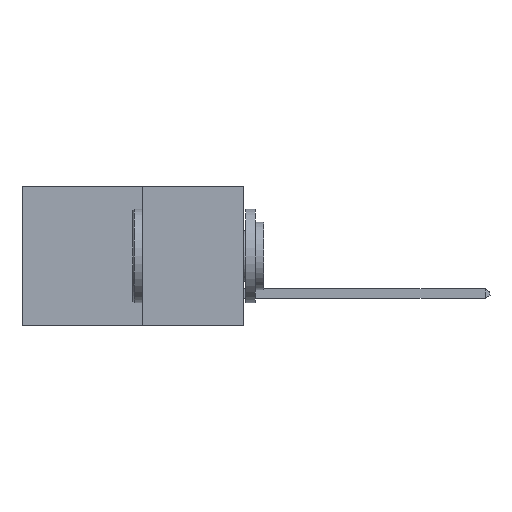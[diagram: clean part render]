
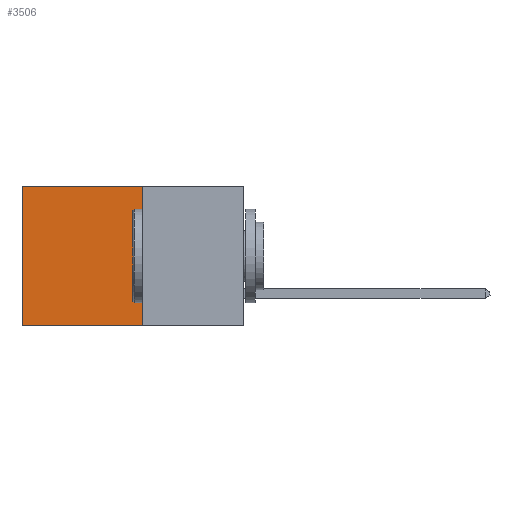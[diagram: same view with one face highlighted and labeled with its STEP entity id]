
A CAD part, left-side view. The second image highlights one B-rep face of the part: STEP entity #3506.
In plain terms, the highlighted planar face has unit normal (-1, 0, 0).
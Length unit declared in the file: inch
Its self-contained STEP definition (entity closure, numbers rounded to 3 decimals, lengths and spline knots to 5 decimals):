
#1034 = LINE ( 'NONE', #5057, #6198 ) ;
#1235 = CARTESIAN_POINT ( 'NONE',  ( 0.277, 0.27, -0.37 ) ) ;
#1250 = PLANE ( 'NONE',  #11223 ) ;
#1860 = LINE ( 'NONE', #7934, #11618 ) ;
#2413 = CARTESIAN_POINT ( 'NONE',  ( 0.277, 0.27, 0. ) ) ;
#3143 = VERTEX_POINT ( 'NONE', #6513 ) ;
#3212 = EDGE_LOOP ( 'NONE', ( #11112, #5758, #11559, #10542 ) ) ;
#3315 = CARTESIAN_POINT ( 'NONE',  ( 0.277, 0.59, 0. ) ) ;
#3506 = ADVANCED_FACE ( 'NONE', ( #8636 ), #1250, .F. ) ;
#3954 = CARTESIAN_POINT ( 'NONE',  ( 0.277, 0.27, -0.37 ) ) ;
#5057 = CARTESIAN_POINT ( 'NONE',  ( 0.277, 0.27, 0. ) ) ;
#5202 = EDGE_CURVE ( 'NONE', #5911, #11133, #1860, .T. ) ;
#5758 = ORIENTED_EDGE ( 'NONE', *, *, #9185, .F. ) ;
#5911 = VERTEX_POINT ( 'NONE', #3315 ) ;
#6198 = VECTOR ( 'NONE', #11553, 39.37008 ) ;
#6513 = CARTESIAN_POINT ( 'NONE',  ( 0.277, 0.27, -0.37 ) ) ;
#7009 = DIRECTION ( 'NONE',  ( 0., 0., -1. ) ) ;
#7519 = LINE ( 'NONE', #1235, #12099 ) ;
#7720 = DIRECTION ( 'NONE',  ( 0., 1., 0. ) ) ;
#7878 = VECTOR ( 'NONE', #7720, 39.37008 ) ;
#7934 = CARTESIAN_POINT ( 'NONE',  ( 0.277, 0.59, -0.37 ) ) ;
#8269 = DIRECTION ( 'NONE',  ( 1., 0., 0. ) ) ;
#8274 = VERTEX_POINT ( 'NONE', #2413 ) ;
#8636 = FACE_OUTER_BOUND ( 'NONE', #3212, .T. ) ;
#9185 = EDGE_CURVE ( 'NONE', #3143, #11133, #10605, .T. ) ;
#9439 = CARTESIAN_POINT ( 'NONE',  ( 0.277, 0.59, -0.37 ) ) ;
#9503 = CARTESIAN_POINT ( 'NONE',  ( 0.277, 0.27, -0.37 ) ) ;
#10542 = ORIENTED_EDGE ( 'NONE', *, *, #11280, .T. ) ;
#10605 = LINE ( 'NONE', #3954, #7878 ) ;
#11112 = ORIENTED_EDGE ( 'NONE', *, *, #5202, .T. ) ;
#11133 = VERTEX_POINT ( 'NONE', #9439 ) ;
#11223 = AXIS2_PLACEMENT_3D ( 'NONE', #9503, #8269, #11912 ) ;
#11280 = EDGE_CURVE ( 'NONE', #8274, #5911, #1034, .T. ) ;
#11379 = EDGE_CURVE ( 'NONE', #8274, #3143, #7519, .T. ) ;
#11553 = DIRECTION ( 'NONE',  ( 0., 1., 0. ) ) ;
#11559 = ORIENTED_EDGE ( 'NONE', *, *, #11379, .F. ) ;
#11618 = VECTOR ( 'NONE', #11627, 39.37008 ) ;
#11627 = DIRECTION ( 'NONE',  ( 0., 0., -1. ) ) ;
#11912 = DIRECTION ( 'NONE',  ( 0., 0., -1. ) ) ;
#12099 = VECTOR ( 'NONE', #7009, 39.37008 ) ;
